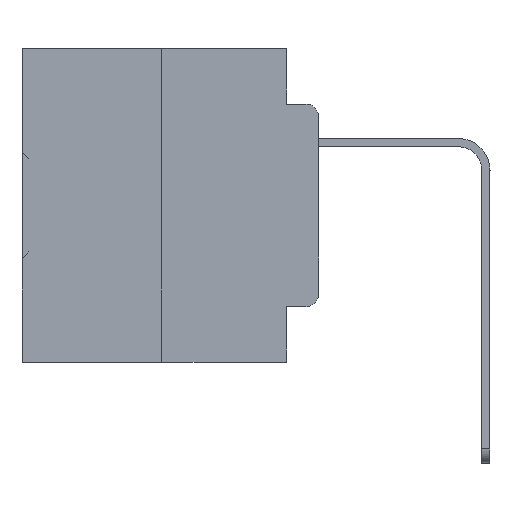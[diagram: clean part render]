
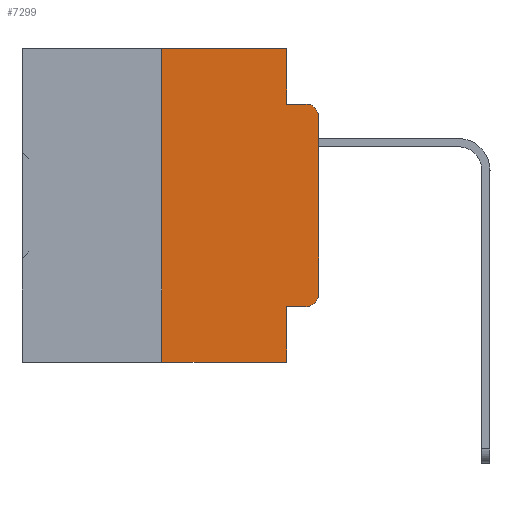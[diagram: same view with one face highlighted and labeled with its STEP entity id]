
A CAD part, left-side view. The second image highlights one B-rep face of the part: STEP entity #7299.
In plain terms, the highlighted planar face has unit normal (-1, 0, 0).
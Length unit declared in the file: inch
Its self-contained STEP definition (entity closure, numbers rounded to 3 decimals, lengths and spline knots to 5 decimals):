
#71 = DIRECTION ( 'NONE',  ( 0., 0., -1. ) ) ;
#438 = CARTESIAN_POINT ( 'NONE',  ( 0., 0.02, -0.0885 ) ) ;
#1194 = LINE ( 'NONE', #2439, #19584 ) ;
#2104 = CARTESIAN_POINT ( 'NONE',  ( 0., 0.051, 0. ) ) ;
#2439 = CARTESIAN_POINT ( 'NONE',  ( 0., 0.051, -0.0885 ) ) ;
#2781 = EDGE_CURVE ( 'NONE', #36938, #11135, #10188, .T. ) ;
#3388 = EDGE_CURVE ( 'NONE', #33494, #27622, #1194, .T. ) ;
#3795 = CARTESIAN_POINT ( 'NONE',  ( 0., 0.25, -0.5 ) ) ;
#3954 = ORIENTED_EDGE ( 'NONE', *, *, #17930, .T. ) ;
#5628 = CARTESIAN_POINT ( 'NONE',  ( 0., 0.473, 0. ) ) ;
#5663 = CARTESIAN_POINT ( 'NONE',  ( 0., 0.473, 0. ) ) ;
#5994 = DIRECTION ( 'NONE',  ( 0., 0., -1. ) ) ;
#6841 = LINE ( 'NONE', #35730, #28869 ) ;
#7299 = ADVANCED_FACE ( 'NONE', ( #13901 ), #37209, .F. ) ;
#7361 = VECTOR ( 'NONE', #20304, 39.37008 ) ;
#8091 = CARTESIAN_POINT ( 'NONE',  ( 0., 0.25, 0. ) ) ;
#8540 = DIRECTION ( 'NONE',  ( 0., 0., -1. ) ) ;
#9089 = VERTEX_POINT ( 'NONE', #17841 ) ;
#9257 = CARTESIAN_POINT ( 'NONE',  ( 0., 0.051, -0.4115 ) ) ;
#10160 = DIRECTION ( 'NONE',  ( 0., 0., 1. ) ) ;
#10188 = LINE ( 'NONE', #16786, #37168 ) ;
#10504 = VECTOR ( 'NONE', #25075, 39.37008 ) ;
#10522 = VECTOR ( 'NONE', #29364, 39.37008 ) ;
#11135 = VERTEX_POINT ( 'NONE', #27640 ) ;
#11906 = CARTESIAN_POINT ( 'NONE',  ( 0., 0., -0.3915 ) ) ;
#12064 = ORIENTED_EDGE ( 'NONE', *, *, #3388, .F. ) ;
#12442 = CARTESIAN_POINT ( 'NONE',  ( 0., 0.051, 0. ) ) ;
#13901 = FACE_OUTER_BOUND ( 'NONE', #29451, .T. ) ;
#14088 = ORIENTED_EDGE ( 'NONE', *, *, #18497, .F. ) ;
#14925 = LINE ( 'NONE', #5628, #25271 ) ;
#15264 = VERTEX_POINT ( 'NONE', #3795 ) ;
#15334 = ORIENTED_EDGE ( 'NONE', *, *, #21883, .T. ) ;
#15653 = CARTESIAN_POINT ( 'NONE',  ( 0., 0.25, 0. ) ) ;
#16006 = EDGE_CURVE ( 'NONE', #15264, #33432, #23272, .T. ) ;
#16153 = ORIENTED_EDGE ( 'NONE', *, *, #16006, .F. ) ;
#16387 = ORIENTED_EDGE ( 'NONE', *, *, #22723, .T. ) ;
#16786 = CARTESIAN_POINT ( 'NONE',  ( 0., 0., 0. ) ) ;
#16811 = LINE ( 'NONE', #9257, #10522 ) ;
#17841 = CARTESIAN_POINT ( 'NONE',  ( 0., 0.051, -0.4115 ) ) ;
#17930 = EDGE_CURVE ( 'NONE', #20967, #36938, #36194, .T. ) ;
#18457 = DIRECTION ( 'NONE',  ( 0., -1., 0. ) ) ;
#18497 = EDGE_CURVE ( 'NONE', #18934, #33494, #27586, .T. ) ;
#18590 = AXIS2_PLACEMENT_3D ( 'NONE', #19872, #23149, #71 ) ;
#18934 = VERTEX_POINT ( 'NONE', #12442 ) ;
#19584 = VECTOR ( 'NONE', #37255, 39.37008 ) ;
#19872 = CARTESIAN_POINT ( 'NONE',  ( 0., 0.02, -0.1085 ) ) ;
#20139 = CARTESIAN_POINT ( 'NONE',  ( 0., 0.02, -0.3915 ) ) ;
#20142 = DIRECTION ( 'NONE',  ( 0., -1., 0. ) ) ;
#20164 = ORIENTED_EDGE ( 'NONE', *, *, #2781, .T. ) ;
#20189 = CARTESIAN_POINT ( 'NONE',  ( 0., 0.051, 0. ) ) ;
#20304 = DIRECTION ( 'NONE',  ( 0., 0., -1. ) ) ;
#20967 = VERTEX_POINT ( 'NONE', #33220 ) ;
#21883 = EDGE_CURVE ( 'NONE', #9089, #20967, #16811, .T. ) ;
#22723 = EDGE_CURVE ( 'NONE', #15264, #28586, #6841, .T. ) ;
#23149 = DIRECTION ( 'NONE',  ( -1., 0., 0. ) ) ;
#23174 = DIRECTION ( 'NONE',  ( -1., 0., 0. ) ) ;
#23272 = LINE ( 'NONE', #15653, #28246 ) ;
#23941 = CARTESIAN_POINT ( 'NONE',  ( 0., 0.051, -0.0885 ) ) ;
#25075 = DIRECTION ( 'NONE',  ( 0., 0., -1. ) ) ;
#25271 = VECTOR ( 'NONE', #20142, 39.37008 ) ;
#25736 = DIRECTION ( 'NONE',  ( 1., 0., 0. ) ) ;
#26549 = ORIENTED_EDGE ( 'NONE', *, *, #28265, .F. ) ;
#26861 = AXIS2_PLACEMENT_3D ( 'NONE', #5663, #25736, #8540 ) ;
#27586 = LINE ( 'NONE', #2104, #10504 ) ;
#27622 = VERTEX_POINT ( 'NONE', #438 ) ;
#27640 = CARTESIAN_POINT ( 'NONE',  ( 0., 0., -0.1085 ) ) ;
#27742 = CARTESIAN_POINT ( 'NONE',  ( 0., 0.051, -0.5 ) ) ;
#28246 = VECTOR ( 'NONE', #10160, 39.37008 ) ;
#28265 = EDGE_CURVE ( 'NONE', #9089, #28586, #28503, .T. ) ;
#28410 = ORIENTED_EDGE ( 'NONE', *, *, #28825, .F. ) ;
#28503 = LINE ( 'NONE', #20189, #7361 ) ;
#28586 = VERTEX_POINT ( 'NONE', #27742 ) ;
#28825 = EDGE_CURVE ( 'NONE', #33432, #18934, #14925, .T. ) ;
#28869 = VECTOR ( 'NONE', #18457, 39.37008 ) ;
#29317 = EDGE_CURVE ( 'NONE', #11135, #27622, #30661, .T. ) ;
#29364 = DIRECTION ( 'NONE',  ( 0., -1., 0. ) ) ;
#29451 = EDGE_LOOP ( 'NONE', ( #20164, #32628, #12064, #14088, #28410, #16153, #16387, #26549, #15334, #3954 ) ) ;
#30661 = CIRCLE ( 'NONE', #18590, 0.02 ) ;
#32516 = AXIS2_PLACEMENT_3D ( 'NONE', #20139, #23174, #5994 ) ;
#32628 = ORIENTED_EDGE ( 'NONE', *, *, #29317, .T. ) ;
#33220 = CARTESIAN_POINT ( 'NONE',  ( 0., 0.02, -0.4115 ) ) ;
#33432 = VERTEX_POINT ( 'NONE', #8091 ) ;
#33494 = VERTEX_POINT ( 'NONE', #23941 ) ;
#34403 = DIRECTION ( 'NONE',  ( 0., 0., 1. ) ) ;
#35730 = CARTESIAN_POINT ( 'NONE',  ( 0., 0.473, -0.5 ) ) ;
#36194 = CIRCLE ( 'NONE', #32516, 0.02 ) ;
#36938 = VERTEX_POINT ( 'NONE', #11906 ) ;
#37168 = VECTOR ( 'NONE', #34403, 39.37008 ) ;
#37209 = PLANE ( 'NONE',  #26861 ) ;
#37255 = DIRECTION ( 'NONE',  ( 0., -1., 0. ) ) ;
